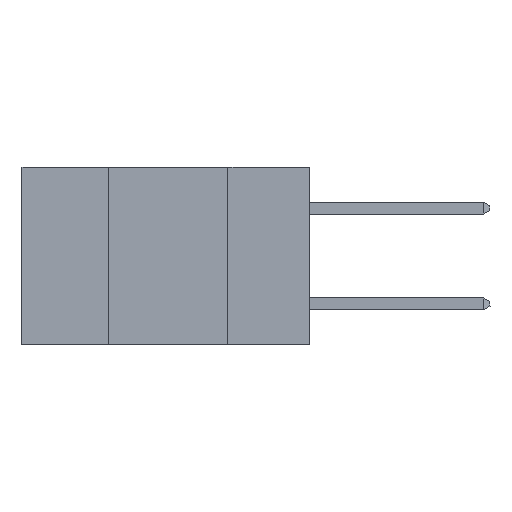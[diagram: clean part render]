
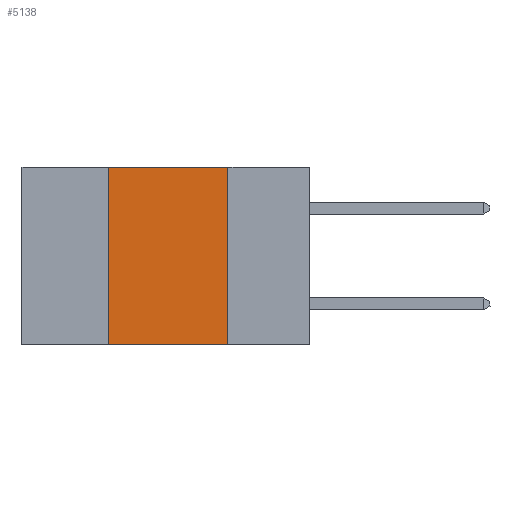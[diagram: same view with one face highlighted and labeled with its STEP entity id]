
A CAD part, left-side view. The second image highlights one B-rep face of the part: STEP entity #5138.
In plain terms, the highlighted planar face has unit normal (-1, 0, 0).
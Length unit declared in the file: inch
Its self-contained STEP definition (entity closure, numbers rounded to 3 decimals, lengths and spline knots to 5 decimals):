
#45 = ORIENTED_EDGE ( 'NONE', *, *, #973, .F. ) ;
#973 = EDGE_CURVE ( 'NONE', #14741, #18555, #8860, .T. ) ;
#1532 = VECTOR ( 'NONE', #6959, 39.37008 ) ;
#1924 = CARTESIAN_POINT ( 'NONE',  ( 0., 0.17, 0. ) ) ;
#2051 = LINE ( 'NONE', #13554, #1532 ) ;
#2146 = ORIENTED_EDGE ( 'NONE', *, *, #3927, .F. ) ;
#2942 = EDGE_CURVE ( 'NONE', #14741, #20838, #7191, .T. ) ;
#3927 = EDGE_CURVE ( 'NONE', #15985, #20838, #4515, .T. ) ;
#4515 = LINE ( 'NONE', #1924, #20915 ) ;
#4518 = AXIS2_PLACEMENT_3D ( 'NONE', #18476, #8683, #20071 ) ;
#5138 = ADVANCED_FACE ( 'NONE', ( #20535 ), #15223, .F. ) ;
#6959 = DIRECTION ( 'NONE',  ( 0., -1., 0. ) ) ;
#7191 = LINE ( 'NONE', #12546, #15424 ) ;
#7416 = DIRECTION ( 'NONE',  ( 0., 0., 1. ) ) ;
#8683 = DIRECTION ( 'NONE',  ( 1., 0., 0. ) ) ;
#8860 = LINE ( 'NONE', #20463, #17011 ) ;
#10927 = CARTESIAN_POINT ( 'NONE',  ( 0., 0.17, -0.37 ) ) ;
#11475 = ORIENTED_EDGE ( 'NONE', *, *, #2942, .T. ) ;
#12546 = CARTESIAN_POINT ( 'NONE',  ( 0., 0.6, -0.37 ) ) ;
#13554 = CARTESIAN_POINT ( 'NONE',  ( 0., 0.6, 0. ) ) ;
#13562 = DIRECTION ( 'NONE',  ( 0., 0., -1. ) ) ;
#13899 = ORIENTED_EDGE ( 'NONE', *, *, #18100, .F. ) ;
#13973 = EDGE_LOOP ( 'NONE', ( #2146, #13899, #45, #11475 ) ) ;
#14202 = DIRECTION ( 'NONE',  ( 0., -1., 0. ) ) ;
#14487 = CARTESIAN_POINT ( 'NONE',  ( 0., 0.42, -0.37 ) ) ;
#14741 = VERTEX_POINT ( 'NONE', #14487 ) ;
#15223 = PLANE ( 'NONE',  #4518 ) ;
#15424 = VECTOR ( 'NONE', #14202, 39.37008 ) ;
#15985 = VERTEX_POINT ( 'NONE', #21081 ) ;
#17011 = VECTOR ( 'NONE', #7416, 39.37008 ) ;
#18100 = EDGE_CURVE ( 'NONE', #18555, #15985, #2051, .T. ) ;
#18476 = CARTESIAN_POINT ( 'NONE',  ( 0., 0.6, 0. ) ) ;
#18555 = VERTEX_POINT ( 'NONE', #19670 ) ;
#19670 = CARTESIAN_POINT ( 'NONE',  ( 0., 0.42, 0. ) ) ;
#20071 = DIRECTION ( 'NONE',  ( 0., 0., -1. ) ) ;
#20463 = CARTESIAN_POINT ( 'NONE',  ( 0., 0.42, 0. ) ) ;
#20535 = FACE_OUTER_BOUND ( 'NONE', #13973, .T. ) ;
#20838 = VERTEX_POINT ( 'NONE', #10927 ) ;
#20915 = VECTOR ( 'NONE', #13562, 39.37008 ) ;
#21081 = CARTESIAN_POINT ( 'NONE',  ( 0., 0.17, 0. ) ) ;
